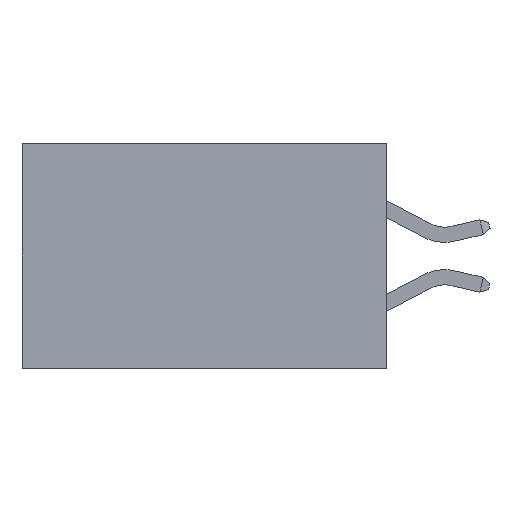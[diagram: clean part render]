
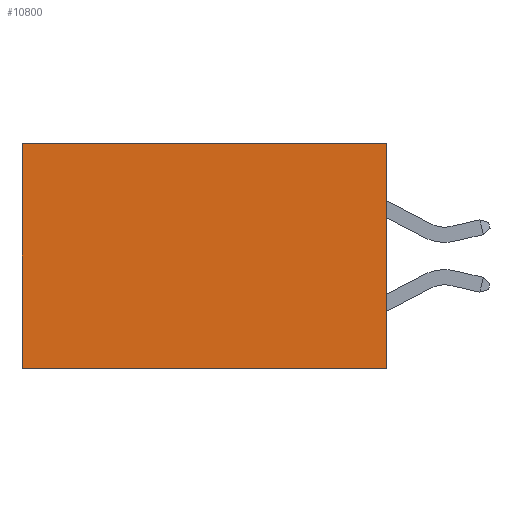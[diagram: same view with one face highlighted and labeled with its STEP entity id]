
A CAD part, left-side view. The second image highlights one B-rep face of the part: STEP entity #10800.
In plain terms, the highlighted planar face has unit normal (-1, 0, 0).
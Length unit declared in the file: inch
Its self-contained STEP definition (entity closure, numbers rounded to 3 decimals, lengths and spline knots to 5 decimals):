
#342 = LINE ( 'NONE', #7480, #11504 ) ;
#564 = FACE_OUTER_BOUND ( 'NONE', #11693, .T. ) ;
#2001 = DIRECTION ( 'NONE',  ( 0., 0., -1. ) ) ;
#2125 = CARTESIAN_POINT ( 'NONE',  ( 0.298, 0., 0. ) ) ;
#2235 = CARTESIAN_POINT ( 'NONE',  ( 0.298, 0.6, 0. ) ) ;
#2591 = CARTESIAN_POINT ( 'NONE',  ( 0.298, 0., 0. ) ) ;
#2619 = LINE ( 'NONE', #5116, #8215 ) ;
#3134 = VECTOR ( 'NONE', #12040, 39.37008 ) ;
#3189 = DIRECTION ( 'NONE',  ( 0., 0., -1. ) ) ;
#3321 = VERTEX_POINT ( 'NONE', #2235 ) ;
#3468 = LINE ( 'NONE', #5763, #3134 ) ;
#4122 = VECTOR ( 'NONE', #2001, 39.37008 ) ;
#4575 = ORIENTED_EDGE ( 'NONE', *, *, #11703, .T. ) ;
#5116 = CARTESIAN_POINT ( 'NONE',  ( 0.298, 0., -0.37 ) ) ;
#5363 = VERTEX_POINT ( 'NONE', #11408 ) ;
#5763 = CARTESIAN_POINT ( 'NONE',  ( 0.298, 0.6, 0. ) ) ;
#7361 = PLANE ( 'NONE',  #12105 ) ;
#7480 = CARTESIAN_POINT ( 'NONE',  ( 0.298, 0., 0. ) ) ;
#8215 = VECTOR ( 'NONE', #11417, 39.37008 ) ;
#9335 = CARTESIAN_POINT ( 'NONE',  ( 0.298, 0., 0. ) ) ;
#9401 = CARTESIAN_POINT ( 'NONE',  ( 0.298, 0., -0.37 ) ) ;
#9503 = DIRECTION ( 'NONE',  ( 1., 0., 0. ) ) ;
#9811 = EDGE_CURVE ( 'NONE', #3321, #5363, #3468, .T. ) ;
#9822 = VERTEX_POINT ( 'NONE', #2591 ) ;
#10037 = EDGE_CURVE ( 'NONE', #11509, #5363, #2619, .T. ) ;
#10090 = EDGE_CURVE ( 'NONE', #9822, #11509, #12492, .T. ) ;
#10800 = ADVANCED_FACE ( 'NONE', ( #564 ), #7361, .F. ) ;
#11027 = ORIENTED_EDGE ( 'NONE', *, *, #9811, .T. ) ;
#11408 = CARTESIAN_POINT ( 'NONE',  ( 0.298, 0.6, -0.37 ) ) ;
#11417 = DIRECTION ( 'NONE',  ( 0., 1., 0. ) ) ;
#11504 = VECTOR ( 'NONE', #12742, 39.37008 ) ;
#11509 = VERTEX_POINT ( 'NONE', #9401 ) ;
#11693 = EDGE_LOOP ( 'NONE', ( #11027, #12293, #12907, #4575 ) ) ;
#11703 = EDGE_CURVE ( 'NONE', #9822, #3321, #342, .T. ) ;
#12040 = DIRECTION ( 'NONE',  ( 0., 0., -1. ) ) ;
#12105 = AXIS2_PLACEMENT_3D ( 'NONE', #2125, #9503, #3189 ) ;
#12293 = ORIENTED_EDGE ( 'NONE', *, *, #10037, .F. ) ;
#12492 = LINE ( 'NONE', #9335, #4122 ) ;
#12742 = DIRECTION ( 'NONE',  ( 0., 1., 0. ) ) ;
#12907 = ORIENTED_EDGE ( 'NONE', *, *, #10090, .F. ) ;
